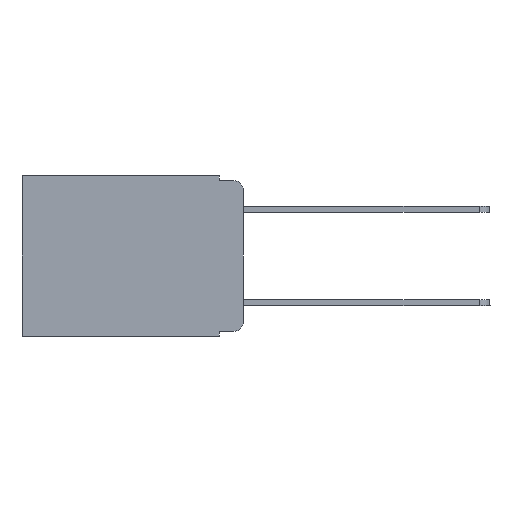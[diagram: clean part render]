
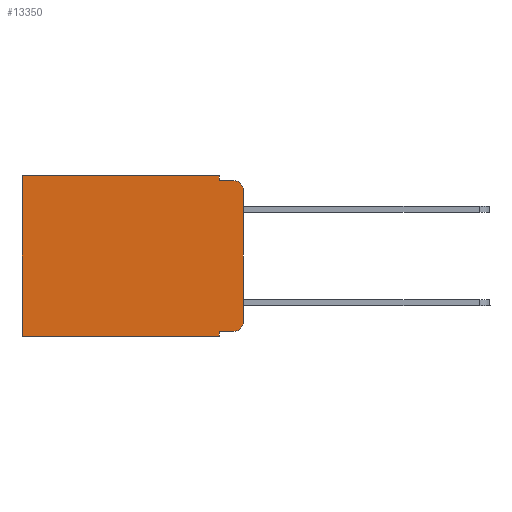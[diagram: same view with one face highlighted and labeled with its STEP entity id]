
A CAD part, left-side view. The second image highlights one B-rep face of the part: STEP entity #13350.
In plain terms, the highlighted planar face has unit normal (-1, 0, 0).
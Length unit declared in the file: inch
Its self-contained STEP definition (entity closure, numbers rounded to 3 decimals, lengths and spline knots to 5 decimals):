
#164 = PLANE ( 'NONE',  #16173 ) ;
#613 = DIRECTION ( 'NONE',  ( -1., 0., 0. ) ) ;
#698 = CARTESIAN_POINT ( 'NONE',  ( 0.298, 0.051, -0.01 ) ) ;
#714 = LINE ( 'NONE', #17536, #11513 ) ;
#955 = DIRECTION ( 'NONE',  ( 0., 0., -1. ) ) ;
#1120 = DIRECTION ( 'NONE',  ( 0., 0., -1. ) ) ;
#1454 = ORIENTED_EDGE ( 'NONE', *, *, #9713, .T. ) ;
#1465 = LINE ( 'NONE', #7941, #13957 ) ;
#1862 = ORIENTED_EDGE ( 'NONE', *, *, #18647, .T. ) ;
#1900 = DIRECTION ( 'NONE',  ( 0., 0., -1. ) ) ;
#2086 = CARTESIAN_POINT ( 'NONE',  ( 0.298, 0., -0.343 ) ) ;
#2283 = DIRECTION ( 'NONE',  ( 0., 0., -1. ) ) ;
#2361 = CARTESIAN_POINT ( 'NONE',  ( 0.298, 0.02, -0.313 ) ) ;
#2491 = DIRECTION ( 'NONE',  ( -1., 0., 0. ) ) ;
#2516 = ORIENTED_EDGE ( 'NONE', *, *, #19207, .T. ) ;
#2779 = EDGE_CURVE ( 'NONE', #10438, #6450, #17157, .T. ) ;
#2948 = CARTESIAN_POINT ( 'NONE',  ( 0.298, 0., -0.313 ) ) ;
#3724 = CARTESIAN_POINT ( 'NONE',  ( 0.298, 0.051, -0.333 ) ) ;
#3740 = EDGE_CURVE ( 'NONE', #20726, #17123, #714, .T. ) ;
#3837 = EDGE_CURVE ( 'NONE', #20726, #14115, #1465, .T. ) ;
#4101 = VERTEX_POINT ( 'NONE', #2948 ) ;
#4841 = EDGE_CURVE ( 'NONE', #13469, #4101, #8958, .T. ) ;
#4983 = VECTOR ( 'NONE', #12700, 39.37008 ) ;
#5371 = DIRECTION ( 'NONE',  ( 0., 0., -1. ) ) ;
#5915 = LINE ( 'NONE', #698, #4983 ) ;
#6386 = ORIENTED_EDGE ( 'NONE', *, *, #4841, .F. ) ;
#6450 = VERTEX_POINT ( 'NONE', #17187 ) ;
#7817 = AXIS2_PLACEMENT_3D ( 'NONE', #2361, #613, #955 ) ;
#7941 = CARTESIAN_POINT ( 'NONE',  ( 0.298, 0., 0. ) ) ;
#8108 = CARTESIAN_POINT ( 'NONE',  ( 0.298, 0.051, -0.343 ) ) ;
#8275 = CARTESIAN_POINT ( 'NONE',  ( 0.298, 0., 0. ) ) ;
#8505 = VERTEX_POINT ( 'NONE', #9924 ) ;
#8836 = EDGE_LOOP ( 'NONE', ( #6386, #2516, #17202, #19685, #21292, #1862, #16823, #16956, #1454, #20054 ) ) ;
#8958 = LINE ( 'NONE', #13946, #14316 ) ;
#9484 = DIRECTION ( 'NONE',  ( 0., -1., 0. ) ) ;
#9713 = EDGE_CURVE ( 'NONE', #15464, #10382, #11057, .T. ) ;
#9924 = CARTESIAN_POINT ( 'NONE',  ( 0.298, 0.02, -0.01 ) ) ;
#10107 = VECTOR ( 'NONE', #13881, 39.37008 ) ;
#10382 = VERTEX_POINT ( 'NONE', #21678 ) ;
#10438 = VERTEX_POINT ( 'NONE', #8108 ) ;
#10543 = VECTOR ( 'NONE', #1120, 39.37008 ) ;
#11057 = LINE ( 'NONE', #16411, #13258 ) ;
#11411 = CIRCLE ( 'NONE', #7817, 0.02 ) ;
#11513 = VECTOR ( 'NONE', #14486, 39.37008 ) ;
#11611 = CARTESIAN_POINT ( 'NONE',  ( 0.298, 0.051, -0.01 ) ) ;
#12338 = EDGE_CURVE ( 'NONE', #15464, #10438, #19582, .T. ) ;
#12700 = DIRECTION ( 'NONE',  ( 0., -1., 0. ) ) ;
#12908 = CARTESIAN_POINT ( 'NONE',  ( 0.298, 0.051, 0. ) ) ;
#13180 = VECTOR ( 'NONE', #5371, 39.37008 ) ;
#13258 = VECTOR ( 'NONE', #9484, 39.37008 ) ;
#13350 = ADVANCED_FACE ( 'NONE', ( #20395 ), #164, .F. ) ;
#13469 = VERTEX_POINT ( 'NONE', #20806 ) ;
#13881 = DIRECTION ( 'NONE',  ( 0., 1., 0. ) ) ;
#13895 = LINE ( 'NONE', #20587, #13180 ) ;
#13946 = CARTESIAN_POINT ( 'NONE',  ( 0.298, 0., 0. ) ) ;
#13957 = VECTOR ( 'NONE', #18413, 39.37008 ) ;
#14115 = VERTEX_POINT ( 'NONE', #18469 ) ;
#14198 = CARTESIAN_POINT ( 'NONE',  ( 0.298, 0.02, -0.03 ) ) ;
#14316 = VECTOR ( 'NONE', #17010, 39.37008 ) ;
#14486 = DIRECTION ( 'NONE',  ( 0., 0., -1. ) ) ;
#14601 = AXIS2_PLACEMENT_3D ( 'NONE', #14198, #2491, #2283 ) ;
#14946 = CIRCLE ( 'NONE', #14601, 0.02 ) ;
#15464 = VERTEX_POINT ( 'NONE', #3724 ) ;
#16173 = AXIS2_PLACEMENT_3D ( 'NONE', #8275, #18410, #1900 ) ;
#16411 = CARTESIAN_POINT ( 'NONE',  ( 0.298, 0.051, -0.333 ) ) ;
#16469 = EDGE_CURVE ( 'NONE', #10382, #4101, #11411, .T. ) ;
#16823 = ORIENTED_EDGE ( 'NONE', *, *, #2779, .F. ) ;
#16886 = EDGE_CURVE ( 'NONE', #17123, #8505, #5915, .T. ) ;
#16956 = ORIENTED_EDGE ( 'NONE', *, *, #12338, .F. ) ;
#17010 = DIRECTION ( 'NONE',  ( 0., 0., -1. ) ) ;
#17123 = VERTEX_POINT ( 'NONE', #11611 ) ;
#17157 = LINE ( 'NONE', #2086, #10107 ) ;
#17187 = CARTESIAN_POINT ( 'NONE',  ( 0.298, 0.473, -0.343 ) ) ;
#17202 = ORIENTED_EDGE ( 'NONE', *, *, #16886, .F. ) ;
#17536 = CARTESIAN_POINT ( 'NONE',  ( 0.298, 0.051, 0. ) ) ;
#18410 = DIRECTION ( 'NONE',  ( 1., 0., 0. ) ) ;
#18413 = DIRECTION ( 'NONE',  ( 0., 1., 0. ) ) ;
#18469 = CARTESIAN_POINT ( 'NONE',  ( 0.298, 0.473, 0. ) ) ;
#18647 = EDGE_CURVE ( 'NONE', #14115, #6450, #13895, .T. ) ;
#18998 = CARTESIAN_POINT ( 'NONE',  ( 0.298, 0.051, 0. ) ) ;
#19207 = EDGE_CURVE ( 'NONE', #13469, #8505, #14946, .T. ) ;
#19582 = LINE ( 'NONE', #12908, #10543 ) ;
#19685 = ORIENTED_EDGE ( 'NONE', *, *, #3740, .F. ) ;
#20054 = ORIENTED_EDGE ( 'NONE', *, *, #16469, .T. ) ;
#20395 = FACE_OUTER_BOUND ( 'NONE', #8836, .T. ) ;
#20587 = CARTESIAN_POINT ( 'NONE',  ( 0.298, 0.473, 0. ) ) ;
#20726 = VERTEX_POINT ( 'NONE', #18998 ) ;
#20806 = CARTESIAN_POINT ( 'NONE',  ( 0.298, 0., -0.03 ) ) ;
#21292 = ORIENTED_EDGE ( 'NONE', *, *, #3837, .T. ) ;
#21678 = CARTESIAN_POINT ( 'NONE',  ( 0.298, 0.02, -0.333 ) ) ;
